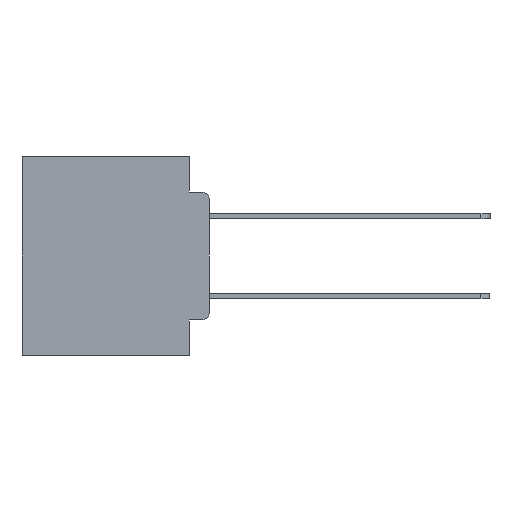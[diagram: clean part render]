
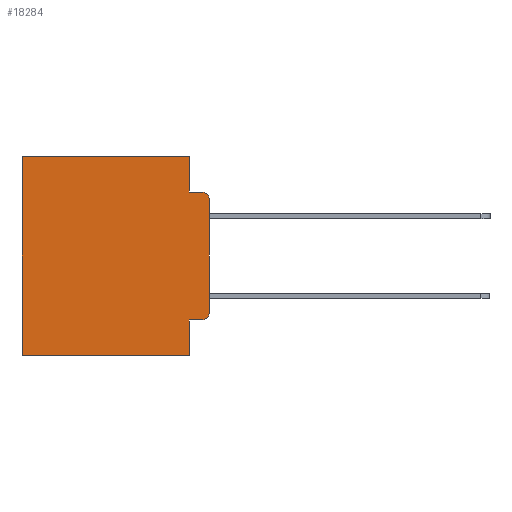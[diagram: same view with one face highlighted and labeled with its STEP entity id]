
A CAD part, left-side view. The second image highlights one B-rep face of the part: STEP entity #18284.
In plain terms, the highlighted planar face has unit normal (-1, 0, 0).
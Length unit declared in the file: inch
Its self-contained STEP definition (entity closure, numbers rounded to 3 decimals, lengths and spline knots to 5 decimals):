
#1116 = EDGE_CURVE ( 'NONE', #7534, #18487, #18658, .T. ) ;
#1330 = DIRECTION ( 'NONE',  ( 0., 0., -1. ) ) ;
#1648 = ORIENTED_EDGE ( 'NONE', *, *, #9143, .T. ) ;
#1776 = VERTEX_POINT ( 'NONE', #12823 ) ;
#2424 = EDGE_CURVE ( 'NONE', #16003, #13876, #11659, .T. ) ;
#2676 = CIRCLE ( 'NONE', #15706, 0.02 ) ;
#3762 = CARTESIAN_POINT ( 'NONE',  ( 0.298, 0.051, 0. ) ) ;
#4071 = DIRECTION ( 'NONE',  ( -1., 0., 0. ) ) ;
#4119 = ORIENTED_EDGE ( 'NONE', *, *, #20442, .T. ) ;
#4780 = CARTESIAN_POINT ( 'NONE',  ( 0.298, 0.051, -0.5 ) ) ;
#5088 = EDGE_LOOP ( 'NONE', ( #19930, #1648, #21925, #16892, #9568, #23861, #26961, #20638, #9142, #4119 ) ) ;
#5495 = VECTOR ( 'NONE', #28343, 39.37008 ) ;
#5531 = LINE ( 'NONE', #22918, #21960 ) ;
#5625 = CARTESIAN_POINT ( 'NONE',  ( 0.298, 0.473, -0.5 ) ) ;
#5787 = VECTOR ( 'NONE', #15964, 39.37008 ) ;
#5806 = VECTOR ( 'NONE', #25163, 39.37008 ) ;
#6442 = VECTOR ( 'NONE', #19476, 39.37008 ) ;
#7534 = VERTEX_POINT ( 'NONE', #25162 ) ;
#7789 = CARTESIAN_POINT ( 'NONE',  ( 0.298, 0., -0.1085 ) ) ;
#8127 = EDGE_CURVE ( 'NONE', #18487, #26446, #5531, .T. ) ;
#8186 = VERTEX_POINT ( 'NONE', #14412 ) ;
#8685 = CARTESIAN_POINT ( 'NONE',  ( 0.298, 0.051, 0. ) ) ;
#9142 = ORIENTED_EDGE ( 'NONE', *, *, #2424, .T. ) ;
#9143 = EDGE_CURVE ( 'NONE', #14005, #8186, #2676, .T. ) ;
#9568 = ORIENTED_EDGE ( 'NONE', *, *, #1116, .T. ) ;
#9725 = DIRECTION ( 'NONE',  ( 0., 0., -1. ) ) ;
#9843 = CARTESIAN_POINT ( 'NONE',  ( 0.298, 0.02, -0.3915 ) ) ;
#10249 = VECTOR ( 'NONE', #16549, 39.37008 ) ;
#11311 = CARTESIAN_POINT ( 'NONE',  ( 0.298, 0., -0.5 ) ) ;
#11363 = FACE_OUTER_BOUND ( 'NONE', #5088, .T. ) ;
#11425 = VERTEX_POINT ( 'NONE', #4780 ) ;
#11523 = CARTESIAN_POINT ( 'NONE',  ( 0.298, 0.051, -0.4115 ) ) ;
#11582 = LINE ( 'NONE', #8685, #5495 ) ;
#11659 = LINE ( 'NONE', #11523, #10249 ) ;
#11763 = AXIS2_PLACEMENT_3D ( 'NONE', #9843, #25153, #12101 ) ;
#11771 = LINE ( 'NONE', #3762, #6442 ) ;
#12101 = DIRECTION ( 'NONE',  ( 0., 0., -1. ) ) ;
#12103 = CARTESIAN_POINT ( 'NONE',  ( 0.298, 0., 0. ) ) ;
#12635 = CARTESIAN_POINT ( 'NONE',  ( 0.298, 0., 0. ) ) ;
#12660 = EDGE_CURVE ( 'NONE', #11425, #26446, #20390, .T. ) ;
#12823 = CARTESIAN_POINT ( 'NONE',  ( 0.298, 0.051, -0.0885 ) ) ;
#13876 = VERTEX_POINT ( 'NONE', #16308 ) ;
#14005 = VERTEX_POINT ( 'NONE', #7789 ) ;
#14180 = AXIS2_PLACEMENT_3D ( 'NONE', #12635, #14878, #1330 ) ;
#14412 = CARTESIAN_POINT ( 'NONE',  ( 0.298, 0.02, -0.0885 ) ) ;
#14592 = EDGE_CURVE ( 'NONE', #14005, #18409, #17780, .T. ) ;
#14878 = DIRECTION ( 'NONE',  ( 1., 0., 0. ) ) ;
#15098 = EDGE_CURVE ( 'NONE', #1776, #8186, #18440, .T. ) ;
#15706 = AXIS2_PLACEMENT_3D ( 'NONE', #17545, #4071, #19772 ) ;
#15964 = DIRECTION ( 'NONE',  ( 0., -1., 0. ) ) ;
#16003 = VERTEX_POINT ( 'NONE', #25368 ) ;
#16308 = CARTESIAN_POINT ( 'NONE',  ( 0.298, 0.02, -0.4115 ) ) ;
#16449 = DIRECTION ( 'NONE',  ( 0., 1., 0. ) ) ;
#16549 = DIRECTION ( 'NONE',  ( 0., -1., 0. ) ) ;
#16892 = ORIENTED_EDGE ( 'NONE', *, *, #28303, .F. ) ;
#17109 = EDGE_CURVE ( 'NONE', #16003, #11425, #11771, .T. ) ;
#17463 = CARTESIAN_POINT ( 'NONE',  ( 0.298, 0., -0.3915 ) ) ;
#17545 = CARTESIAN_POINT ( 'NONE',  ( 0.298, 0.02, -0.1085 ) ) ;
#17780 = LINE ( 'NONE', #23136, #5806 ) ;
#18284 = ADVANCED_FACE ( 'NONE', ( #11363 ), #25665, .F. ) ;
#18409 = VERTEX_POINT ( 'NONE', #17463 ) ;
#18440 = LINE ( 'NONE', #22470, #5787 ) ;
#18487 = VERTEX_POINT ( 'NONE', #19984 ) ;
#18658 = LINE ( 'NONE', #12103, #23721 ) ;
#19476 = DIRECTION ( 'NONE',  ( 0., 0., -1. ) ) ;
#19772 = DIRECTION ( 'NONE',  ( 0., 0., -1. ) ) ;
#19930 = ORIENTED_EDGE ( 'NONE', *, *, #14592, .F. ) ;
#19984 = CARTESIAN_POINT ( 'NONE',  ( 0.298, 0.473, 0. ) ) ;
#20220 = DIRECTION ( 'NONE',  ( 0., 1., 0. ) ) ;
#20390 = LINE ( 'NONE', #11311, #24706 ) ;
#20442 = EDGE_CURVE ( 'NONE', #13876, #18409, #22161, .T. ) ;
#20638 = ORIENTED_EDGE ( 'NONE', *, *, #17109, .F. ) ;
#21925 = ORIENTED_EDGE ( 'NONE', *, *, #15098, .F. ) ;
#21960 = VECTOR ( 'NONE', #9725, 39.37008 ) ;
#22161 = CIRCLE ( 'NONE', #11763, 0.02 ) ;
#22470 = CARTESIAN_POINT ( 'NONE',  ( 0.298, 0.051, -0.0885 ) ) ;
#22918 = CARTESIAN_POINT ( 'NONE',  ( 0.298, 0.473, 0. ) ) ;
#23136 = CARTESIAN_POINT ( 'NONE',  ( 0.298, 0., 0. ) ) ;
#23721 = VECTOR ( 'NONE', #16449, 39.37008 ) ;
#23861 = ORIENTED_EDGE ( 'NONE', *, *, #8127, .T. ) ;
#24706 = VECTOR ( 'NONE', #20220, 39.37008 ) ;
#25153 = DIRECTION ( 'NONE',  ( -1., 0., 0. ) ) ;
#25162 = CARTESIAN_POINT ( 'NONE',  ( 0.298, 0.051, 0. ) ) ;
#25163 = DIRECTION ( 'NONE',  ( 0., 0., -1. ) ) ;
#25368 = CARTESIAN_POINT ( 'NONE',  ( 0.298, 0.051, -0.4115 ) ) ;
#25665 = PLANE ( 'NONE',  #14180 ) ;
#26446 = VERTEX_POINT ( 'NONE', #5625 ) ;
#26961 = ORIENTED_EDGE ( 'NONE', *, *, #12660, .F. ) ;
#28303 = EDGE_CURVE ( 'NONE', #7534, #1776, #11582, .T. ) ;
#28343 = DIRECTION ( 'NONE',  ( 0., 0., -1. ) ) ;
